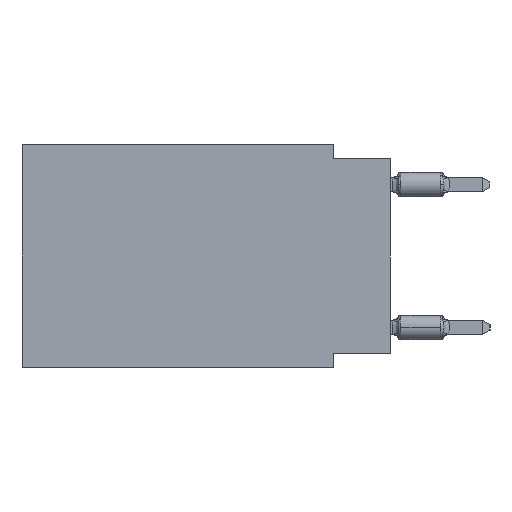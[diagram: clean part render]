
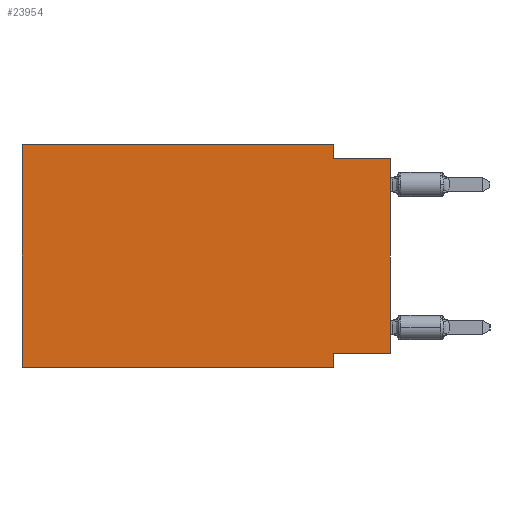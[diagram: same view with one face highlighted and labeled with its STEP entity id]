
A CAD part, left-side view. The second image highlights one B-rep face of the part: STEP entity #23954.
In plain terms, the highlighted planar face has unit normal (-1, 0, 0).
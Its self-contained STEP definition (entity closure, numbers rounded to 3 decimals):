
#565 = CARTESIAN_POINT ( 'NONE',  ( 0., 16.383, -9.906 ) ) ;
#1396 = EDGE_CURVE ( 'NONE', #31359, #21482, #28600, .T. ) ;
#2392 = ORIENTED_EDGE ( 'NONE', *, *, #3099, .T. ) ;
#2737 = EDGE_CURVE ( 'NONE', #9738, #25610, #6082, .T. ) ;
#3099 = EDGE_CURVE ( 'NONE', #12844, #23009, #25398, .T. ) ;
#3278 = ORIENTED_EDGE ( 'NONE', *, *, #4025, .F. ) ;
#3781 = VECTOR ( 'NONE', #30757, 1000. ) ;
#4025 = EDGE_CURVE ( 'NONE', #19493, #23009, #25219, .T. ) ;
#4390 = VECTOR ( 'NONE', #17092, 1000. ) ;
#4793 = EDGE_CURVE ( 'NONE', #20102, #31359, #8154, .T. ) ;
#4833 = EDGE_CURVE ( 'NONE', #20102, #25610, #11475, .T. ) ;
#5484 = PLANE ( 'NONE',  #23945 ) ;
#6082 = LINE ( 'NONE', #25808, #9028 ) ;
#7679 = CARTESIAN_POINT ( 'NONE',  ( 0., 2.54, -0.635 ) ) ;
#8154 = LINE ( 'NONE', #25645, #4390 ) ;
#8506 = VECTOR ( 'NONE', #30994, 1000. ) ;
#8825 = CARTESIAN_POINT ( 'NONE',  ( 0., 0., 0. ) ) ;
#9028 = VECTOR ( 'NONE', #31947, 1000. ) ;
#9172 = CARTESIAN_POINT ( 'NONE',  ( 0., 16.383, 0. ) ) ;
#9738 = VERTEX_POINT ( 'NONE', #18381 ) ;
#10727 = ORIENTED_EDGE ( 'NONE', *, *, #23792, .F. ) ;
#10806 = ORIENTED_EDGE ( 'NONE', *, *, #24649, .F. ) ;
#11022 = ORIENTED_EDGE ( 'NONE', *, *, #4793, .F. ) ;
#11237 = FACE_OUTER_BOUND ( 'NONE', #30366, .T. ) ;
#11475 = LINE ( 'NONE', #25085, #36477 ) ;
#12127 = CARTESIAN_POINT ( 'NONE',  ( 0., 0., -0.635 ) ) ;
#12844 = VERTEX_POINT ( 'NONE', #30958 ) ;
#14219 = DIRECTION ( 'NONE',  ( 1., 0., 0. ) ) ;
#14590 = DIRECTION ( 'NONE',  ( 0., 0., -1. ) ) ;
#17092 = DIRECTION ( 'NONE',  ( 0., 0., 1. ) ) ;
#17165 = ORIENTED_EDGE ( 'NONE', *, *, #2737, .F. ) ;
#17203 = DIRECTION ( 'NONE',  ( 0., 0., 1. ) ) ;
#18381 = CARTESIAN_POINT ( 'NONE',  ( 0., 2.54, -9.271 ) ) ;
#18612 = VECTOR ( 'NONE', #26724, 1000. ) ;
#19493 = VERTEX_POINT ( 'NONE', #7679 ) ;
#20102 = VERTEX_POINT ( 'NONE', #565 ) ;
#20244 = DIRECTION ( 'NONE',  ( 0., -1., 0. ) ) ;
#20840 = VECTOR ( 'NONE', #20244, 1000. ) ;
#21341 = LINE ( 'NONE', #29509, #18612 ) ;
#21482 = VERTEX_POINT ( 'NONE', #33965 ) ;
#21560 = VECTOR ( 'NONE', #17203, 1000. ) ;
#23009 = VERTEX_POINT ( 'NONE', #12127 ) ;
#23026 = CARTESIAN_POINT ( 'NONE',  ( 0., 16.383, 0. ) ) ;
#23792 = EDGE_CURVE ( 'NONE', #21482, #19493, #21341, .T. ) ;
#23945 = AXIS2_PLACEMENT_3D ( 'NONE', #9172, #14219, #14590 ) ;
#23954 = ADVANCED_FACE ( 'NONE', ( #11237 ), #5484, .F. ) ;
#24649 = EDGE_CURVE ( 'NONE', #12844, #9738, #24967, .T. ) ;
#24967 = LINE ( 'NONE', #25709, #3781 ) ;
#25085 = CARTESIAN_POINT ( 'NONE',  ( 0., 16.383, -9.906 ) ) ;
#25219 = LINE ( 'NONE', #34163, #8506 ) ;
#25398 = LINE ( 'NONE', #8825, #21560 ) ;
#25610 = VERTEX_POINT ( 'NONE', #25962 ) ;
#25645 = CARTESIAN_POINT ( 'NONE',  ( 0., 16.383, 0. ) ) ;
#25709 = CARTESIAN_POINT ( 'NONE',  ( 0., 0., -9.271 ) ) ;
#25808 = CARTESIAN_POINT ( 'NONE',  ( 0., 2.54, -9.906 ) ) ;
#25962 = CARTESIAN_POINT ( 'NONE',  ( 0., 2.54, -9.906 ) ) ;
#26724 = DIRECTION ( 'NONE',  ( 0., 0., -1. ) ) ;
#28600 = LINE ( 'NONE', #23026, #20840 ) ;
#29509 = CARTESIAN_POINT ( 'NONE',  ( 0., 2.54, 0. ) ) ;
#30366 = EDGE_LOOP ( 'NONE', ( #2392, #3278, #10727, #35257, #11022, #35580, #17165, #10806 ) ) ;
#30675 = CARTESIAN_POINT ( 'NONE',  ( 0., 16.383, 0. ) ) ;
#30757 = DIRECTION ( 'NONE',  ( 0., 1., 0. ) ) ;
#30958 = CARTESIAN_POINT ( 'NONE',  ( 0., 0., -9.271 ) ) ;
#30994 = DIRECTION ( 'NONE',  ( 0., -1., 0. ) ) ;
#31359 = VERTEX_POINT ( 'NONE', #30675 ) ;
#31947 = DIRECTION ( 'NONE',  ( 0., 0., -1. ) ) ;
#33965 = CARTESIAN_POINT ( 'NONE',  ( 0., 2.54, 0. ) ) ;
#34163 = CARTESIAN_POINT ( 'NONE',  ( 0., 0., -0.635 ) ) ;
#35257 = ORIENTED_EDGE ( 'NONE', *, *, #1396, .F. ) ;
#35580 = ORIENTED_EDGE ( 'NONE', *, *, #4833, .T. ) ;
#36436 = DIRECTION ( 'NONE',  ( 0., -1., 0. ) ) ;
#36477 = VECTOR ( 'NONE', #36436, 1000. ) ;
